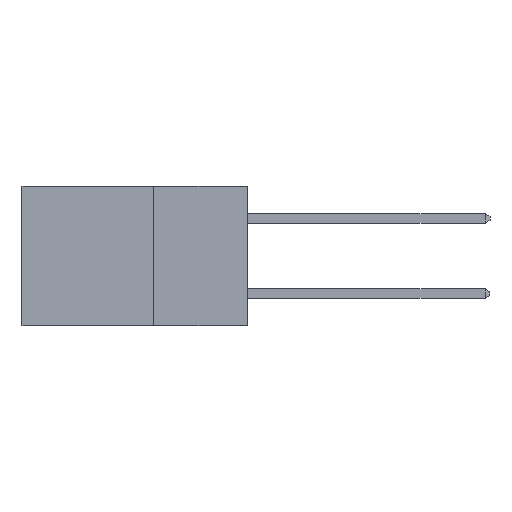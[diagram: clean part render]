
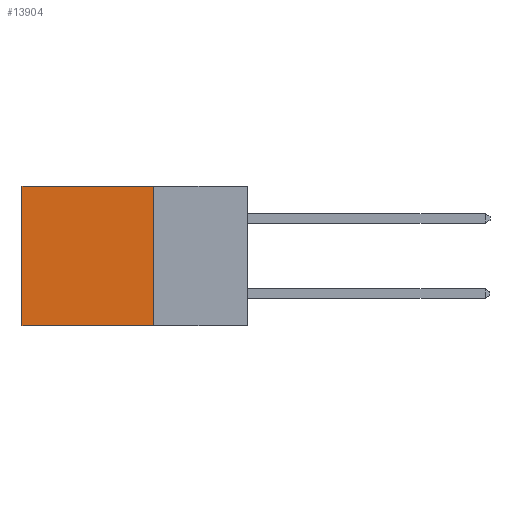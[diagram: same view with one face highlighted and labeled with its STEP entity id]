
A CAD part, left-side view. The second image highlights one B-rep face of the part: STEP entity #13904.
In plain terms, the highlighted planar face has unit normal (-1, 0, 0).
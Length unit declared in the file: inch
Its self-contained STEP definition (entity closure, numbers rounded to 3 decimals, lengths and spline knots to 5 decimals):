
#223 = LINE ( 'NONE', #1290, #9713 ) ;
#250 = ORIENTED_EDGE ( 'NONE', *, *, #9788, .T. ) ;
#807 = DIRECTION ( 'NONE',  ( 0., 0., -1. ) ) ;
#1290 = CARTESIAN_POINT ( 'NONE',  ( 0.298, 0.25, -0.37 ) ) ;
#1377 = VERTEX_POINT ( 'NONE', #2633 ) ;
#1673 = PLANE ( 'NONE',  #2632 ) ;
#1716 = VECTOR ( 'NONE', #12930, 39.37008 ) ;
#2538 = LINE ( 'NONE', #9438, #9460 ) ;
#2632 = AXIS2_PLACEMENT_3D ( 'NONE', #4068, #10268, #2910 ) ;
#2633 = CARTESIAN_POINT ( 'NONE',  ( 0.298, 0.25, 0. ) ) ;
#2910 = DIRECTION ( 'NONE',  ( 0., 0., -1. ) ) ;
#3511 = ORIENTED_EDGE ( 'NONE', *, *, #7736, .F. ) ;
#4068 = CARTESIAN_POINT ( 'NONE',  ( 0.298, 0.25, 0. ) ) ;
#4416 = ORIENTED_EDGE ( 'NONE', *, *, #12384, .F. ) ;
#4599 = ORIENTED_EDGE ( 'NONE', *, *, #11379, .T. ) ;
#6162 = VERTEX_POINT ( 'NONE', #11335 ) ;
#6465 = VECTOR ( 'NONE', #12287, 39.37008 ) ;
#6725 = VERTEX_POINT ( 'NONE', #14624 ) ;
#7736 = EDGE_CURVE ( 'NONE', #1377, #12030, #2538, .T. ) ;
#9079 = FACE_OUTER_BOUND ( 'NONE', #14563, .T. ) ;
#9438 = CARTESIAN_POINT ( 'NONE',  ( 0.298, 0.25, 0. ) ) ;
#9460 = VECTOR ( 'NONE', #807, 39.37008 ) ;
#9713 = VECTOR ( 'NONE', #12209, 39.37008 ) ;
#9753 = LINE ( 'NONE', #11046, #6465 ) ;
#9788 = EDGE_CURVE ( 'NONE', #6162, #6725, #11440, .T. ) ;
#10268 = DIRECTION ( 'NONE',  ( 1., 0., 0. ) ) ;
#11046 = CARTESIAN_POINT ( 'NONE',  ( 0.298, 0.25, 0. ) ) ;
#11335 = CARTESIAN_POINT ( 'NONE',  ( 0.298, 0.6, 0. ) ) ;
#11379 = EDGE_CURVE ( 'NONE', #1377, #6162, #9753, .T. ) ;
#11440 = LINE ( 'NONE', #11748, #1716 ) ;
#11748 = CARTESIAN_POINT ( 'NONE',  ( 0.298, 0.6, 0. ) ) ;
#12030 = VERTEX_POINT ( 'NONE', #14681 ) ;
#12209 = DIRECTION ( 'NONE',  ( 0., 1., 0. ) ) ;
#12287 = DIRECTION ( 'NONE',  ( 0., 1., 0. ) ) ;
#12384 = EDGE_CURVE ( 'NONE', #12030, #6725, #223, .T. ) ;
#12930 = DIRECTION ( 'NONE',  ( 0., 0., -1. ) ) ;
#13904 = ADVANCED_FACE ( 'NONE', ( #9079 ), #1673, .F. ) ;
#14563 = EDGE_LOOP ( 'NONE', ( #250, #4416, #3511, #4599 ) ) ;
#14624 = CARTESIAN_POINT ( 'NONE',  ( 0.298, 0.6, -0.37 ) ) ;
#14681 = CARTESIAN_POINT ( 'NONE',  ( 0.298, 0.25, -0.37 ) ) ;
